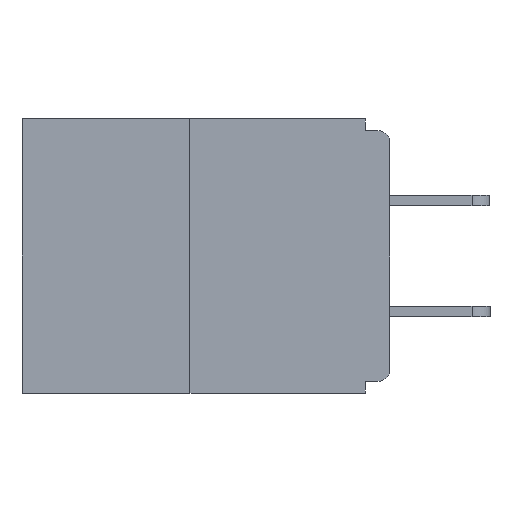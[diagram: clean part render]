
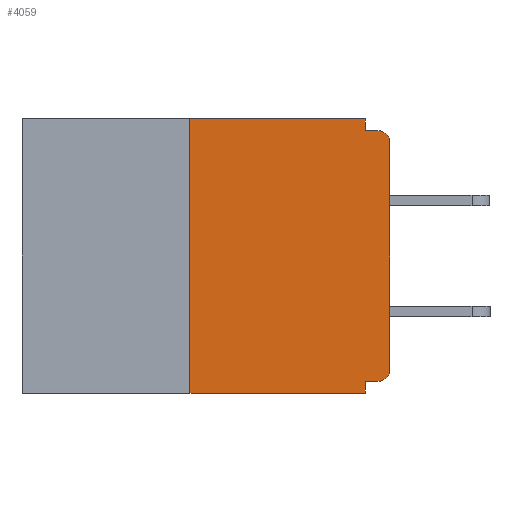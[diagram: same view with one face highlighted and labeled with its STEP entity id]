
A CAD part, left-side view. The second image highlights one B-rep face of the part: STEP entity #4059.
In plain terms, the highlighted planar face has unit normal (-1, 0, 0).
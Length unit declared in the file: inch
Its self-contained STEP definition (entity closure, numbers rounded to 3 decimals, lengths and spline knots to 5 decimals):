
#48 = DIRECTION ( 'NONE',  ( -1., 0., 0. ) ) ;
#131 = CARTESIAN_POINT ( 'NONE',  ( 0., 0., 0. ) ) ;
#390 = LINE ( 'NONE', #7996, #8778 ) ;
#648 = VECTOR ( 'NONE', #4772, 39.37008 ) ;
#965 = EDGE_CURVE ( 'NONE', #9633, #9797, #10468, .T. ) ;
#1004 = LINE ( 'NONE', #7367, #12834 ) ;
#1083 = AXIS2_PLACEMENT_3D ( 'NONE', #14826, #2235, #4543 ) ;
#1113 = CIRCLE ( 'NONE', #10352, 0.015 ) ;
#1770 = DIRECTION ( 'NONE',  ( 0., 0., 1. ) ) ;
#2235 = DIRECTION ( 'NONE',  ( -1., 0., 0. ) ) ;
#2313 = CARTESIAN_POINT ( 'NONE',  ( 0., 0.015, -0.03 ) ) ;
#3279 = CARTESIAN_POINT ( 'NONE',  ( 0., 0.031, -0.328 ) ) ;
#3558 = CARTESIAN_POINT ( 'NONE',  ( 0., 0.031, 0. ) ) ;
#3775 = EDGE_CURVE ( 'NONE', #4074, #9171, #13791, .T. ) ;
#3785 = VERTEX_POINT ( 'NONE', #10527 ) ;
#3934 = EDGE_CURVE ( 'NONE', #14267, #9633, #4855, .T. ) ;
#4059 = ADVANCED_FACE ( 'NONE', ( #14350 ), #13553, .F. ) ;
#4061 = CARTESIAN_POINT ( 'NONE',  ( 0., 0., -0.328 ) ) ;
#4074 = VERTEX_POINT ( 'NONE', #7972 ) ;
#4087 = EDGE_CURVE ( 'NONE', #9797, #7216, #12549, .T. ) ;
#4394 = DIRECTION ( 'NONE',  ( 1., 0., 0. ) ) ;
#4537 = DIRECTION ( 'NONE',  ( 0., 0., -1. ) ) ;
#4543 = DIRECTION ( 'NONE',  ( 0., 0., -1. ) ) ;
#4772 = DIRECTION ( 'NONE',  ( 0., 0., -1. ) ) ;
#4855 = LINE ( 'NONE', #7110, #8052 ) ;
#5074 = EDGE_CURVE ( 'NONE', #13242, #14267, #1004, .T. ) ;
#5137 = CARTESIAN_POINT ( 'NONE',  ( 0., 0.031, -0.015 ) ) ;
#5479 = CARTESIAN_POINT ( 'NONE',  ( 0., 0.015, -0.328 ) ) ;
#5484 = CARTESIAN_POINT ( 'NONE',  ( 0., 0., -0.015 ) ) ;
#5585 = DIRECTION ( 'NONE',  ( 0., -1., 0. ) ) ;
#6362 = DIRECTION ( 'NONE',  ( 0., -1., 0. ) ) ;
#6592 = EDGE_LOOP ( 'NONE', ( #12540, #7530, #10088, #7630, #11095, #14227, #7927, #12928, #12047, #10498 ) ) ;
#6699 = EDGE_CURVE ( 'NONE', #13914, #3785, #8098, .T. ) ;
#7086 = EDGE_CURVE ( 'NONE', #9978, #13914, #11516, .T. ) ;
#7110 = CARTESIAN_POINT ( 'NONE',  ( 0., 0.46, 0. ) ) ;
#7216 = VERTEX_POINT ( 'NONE', #12440 ) ;
#7367 = CARTESIAN_POINT ( 'NONE',  ( 0., 0.25, 0. ) ) ;
#7373 = VECTOR ( 'NONE', #14388, 39.37008 ) ;
#7530 = ORIENTED_EDGE ( 'NONE', *, *, #5074, .F. ) ;
#7630 = ORIENTED_EDGE ( 'NONE', *, *, #6699, .F. ) ;
#7927 = ORIENTED_EDGE ( 'NONE', *, *, #3775, .T. ) ;
#7972 = CARTESIAN_POINT ( 'NONE',  ( 0., 0., -0.313 ) ) ;
#7996 = CARTESIAN_POINT ( 'NONE',  ( 0., 0.46, -0.343 ) ) ;
#8052 = VECTOR ( 'NONE', #6362, 39.37008 ) ;
#8098 = LINE ( 'NONE', #11384, #13840 ) ;
#8778 = VECTOR ( 'NONE', #12528, 39.37008 ) ;
#8927 = DIRECTION ( 'NONE',  ( 0., 0., -1. ) ) ;
#9171 = VERTEX_POINT ( 'NONE', #10908 ) ;
#9476 = EDGE_CURVE ( 'NONE', #9171, #7216, #1113, .T. ) ;
#9633 = VERTEX_POINT ( 'NONE', #12897 ) ;
#9797 = VERTEX_POINT ( 'NONE', #5137 ) ;
#9943 = CARTESIAN_POINT ( 'NONE',  ( 0., 0.25, -0.343 ) ) ;
#9978 = VERTEX_POINT ( 'NONE', #5479 ) ;
#10088 = ORIENTED_EDGE ( 'NONE', *, *, #10749, .T. ) ;
#10352 = AXIS2_PLACEMENT_3D ( 'NONE', #2313, #48, #4537 ) ;
#10468 = LINE ( 'NONE', #3558, #648 ) ;
#10473 = DIRECTION ( 'NONE',  ( 0., 0., 1. ) ) ;
#10498 = ORIENTED_EDGE ( 'NONE', *, *, #965, .F. ) ;
#10527 = CARTESIAN_POINT ( 'NONE',  ( 0., 0.031, -0.343 ) ) ;
#10749 = EDGE_CURVE ( 'NONE', #13242, #3785, #390, .T. ) ;
#10908 = CARTESIAN_POINT ( 'NONE',  ( 0., 0., -0.03 ) ) ;
#11095 = ORIENTED_EDGE ( 'NONE', *, *, #7086, .F. ) ;
#11308 = VECTOR ( 'NONE', #5585, 39.37008 ) ;
#11309 = CIRCLE ( 'NONE', #1083, 0.015 ) ;
#11384 = CARTESIAN_POINT ( 'NONE',  ( 0., 0.031, -0.343 ) ) ;
#11403 = CARTESIAN_POINT ( 'NONE',  ( 0., 0.25, 0. ) ) ;
#11516 = LINE ( 'NONE', #4061, #7373 ) ;
#12047 = ORIENTED_EDGE ( 'NONE', *, *, #4087, .F. ) ;
#12440 = CARTESIAN_POINT ( 'NONE',  ( 0., 0.015, -0.015 ) ) ;
#12498 = EDGE_CURVE ( 'NONE', #9978, #4074, #11309, .T. ) ;
#12528 = DIRECTION ( 'NONE',  ( 0., -1., 0. ) ) ;
#12537 = DIRECTION ( 'NONE',  ( 0., 0., -1. ) ) ;
#12540 = ORIENTED_EDGE ( 'NONE', *, *, #3934, .F. ) ;
#12548 = CARTESIAN_POINT ( 'NONE',  ( 0., 0.46, 0. ) ) ;
#12549 = LINE ( 'NONE', #5484, #11308 ) ;
#12834 = VECTOR ( 'NONE', #1770, 39.37008 ) ;
#12897 = CARTESIAN_POINT ( 'NONE',  ( 0., 0.031, 0. ) ) ;
#12918 = VECTOR ( 'NONE', #10473, 39.37008 ) ;
#12928 = ORIENTED_EDGE ( 'NONE', *, *, #9476, .T. ) ;
#13242 = VERTEX_POINT ( 'NONE', #9943 ) ;
#13553 = PLANE ( 'NONE',  #14454 ) ;
#13791 = LINE ( 'NONE', #131, #12918 ) ;
#13840 = VECTOR ( 'NONE', #12537, 39.37008 ) ;
#13914 = VERTEX_POINT ( 'NONE', #3279 ) ;
#14227 = ORIENTED_EDGE ( 'NONE', *, *, #12498, .T. ) ;
#14267 = VERTEX_POINT ( 'NONE', #11403 ) ;
#14350 = FACE_OUTER_BOUND ( 'NONE', #6592, .T. ) ;
#14388 = DIRECTION ( 'NONE',  ( 0., 1., 0. ) ) ;
#14454 = AXIS2_PLACEMENT_3D ( 'NONE', #12548, #4394, #8927 ) ;
#14826 = CARTESIAN_POINT ( 'NONE',  ( 0., 0.015, -0.313 ) ) ;
